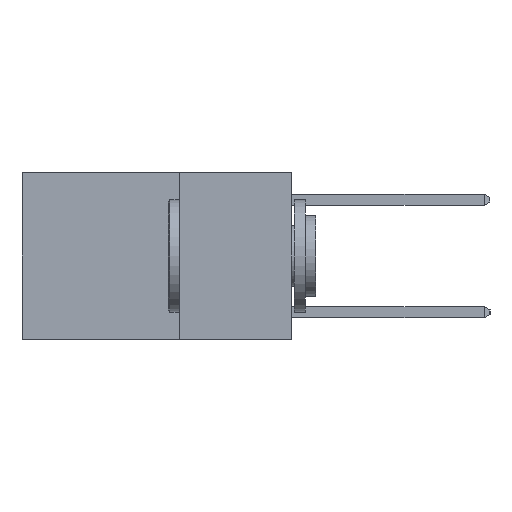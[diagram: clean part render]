
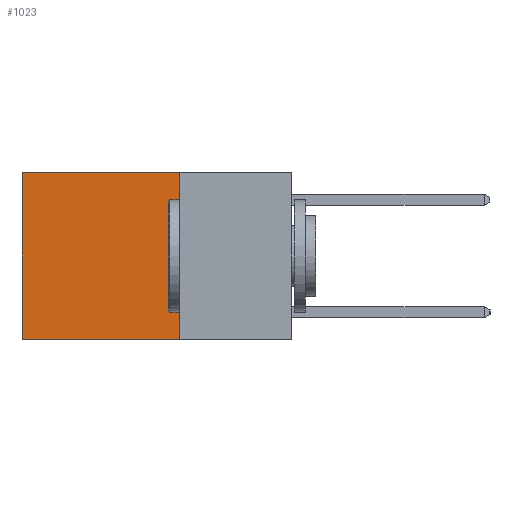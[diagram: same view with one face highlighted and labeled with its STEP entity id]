
A CAD part, left-side view. The second image highlights one B-rep face of the part: STEP entity #1023.
In plain terms, the highlighted planar face has unit normal (-1, 0, 0).
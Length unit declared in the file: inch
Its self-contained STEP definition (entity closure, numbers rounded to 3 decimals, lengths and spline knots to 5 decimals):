
#367 = VECTOR ( 'NONE', #6988, 39.37008 ) ;
#983 = ORIENTED_EDGE ( 'NONE', *, *, #10820, .F. ) ;
#1023 = ADVANCED_FACE ( 'NONE', ( #6357 ), #8432, .F. ) ;
#1138 = DIRECTION ( 'NONE',  ( 0., 0., -1. ) ) ;
#1522 = ORIENTED_EDGE ( 'NONE', *, *, #5323, .F. ) ;
#1647 = CARTESIAN_POINT ( 'NONE',  ( 0.2625, 0.6, -0.37 ) ) ;
#1704 = CARTESIAN_POINT ( 'NONE',  ( 0.2625, 0.6, 0. ) ) ;
#1836 = ORIENTED_EDGE ( 'NONE', *, *, #4123, .T. ) ;
#2904 = CARTESIAN_POINT ( 'NONE',  ( 0.2625, 0.25, 0. ) ) ;
#3054 = CARTESIAN_POINT ( 'NONE',  ( 0.2625, 0.25, 0. ) ) ;
#3218 = VERTEX_POINT ( 'NONE', #5311 ) ;
#3484 = EDGE_LOOP ( 'NONE', ( #4224, #1522, #983, #1836 ) ) ;
#3866 = VECTOR ( 'NONE', #6469, 39.37008 ) ;
#3881 = DIRECTION ( 'NONE',  ( 0., 1., 0. ) ) ;
#4123 = EDGE_CURVE ( 'NONE', #6299, #9887, #9869, .T. ) ;
#4142 = LINE ( 'NONE', #10705, #3866 ) ;
#4224 = ORIENTED_EDGE ( 'NONE', *, *, #5061, .T. ) ;
#4277 = LINE ( 'NONE', #4432, #367 ) ;
#4432 = CARTESIAN_POINT ( 'NONE',  ( 0.2625, 0.6, 0. ) ) ;
#5061 = EDGE_CURVE ( 'NONE', #9887, #5654, #4277, .T. ) ;
#5122 = DIRECTION ( 'NONE',  ( 0., 0., -1. ) ) ;
#5311 = CARTESIAN_POINT ( 'NONE',  ( 0.2625, 0.25, -0.37 ) ) ;
#5323 = EDGE_CURVE ( 'NONE', #3218, #5654, #4142, .T. ) ;
#5654 = VERTEX_POINT ( 'NONE', #1647 ) ;
#6299 = VERTEX_POINT ( 'NONE', #3054 ) ;
#6340 = CARTESIAN_POINT ( 'NONE',  ( 0.2625, 0.25, 0. ) ) ;
#6357 = FACE_OUTER_BOUND ( 'NONE', #3484, .T. ) ;
#6469 = DIRECTION ( 'NONE',  ( 0., 1., 0. ) ) ;
#6988 = DIRECTION ( 'NONE',  ( 0., 0., -1. ) ) ;
#7367 = LINE ( 'NONE', #6340, #9063 ) ;
#7979 = AXIS2_PLACEMENT_3D ( 'NONE', #2904, #9110, #5122 ) ;
#8432 = PLANE ( 'NONE',  #7979 ) ;
#9063 = VECTOR ( 'NONE', #1138, 39.37008 ) ;
#9110 = DIRECTION ( 'NONE',  ( 1., 0., 0. ) ) ;
#9585 = VECTOR ( 'NONE', #3881, 39.37008 ) ;
#9811 = CARTESIAN_POINT ( 'NONE',  ( 0.2625, 0.25, 0. ) ) ;
#9869 = LINE ( 'NONE', #9811, #9585 ) ;
#9887 = VERTEX_POINT ( 'NONE', #1704 ) ;
#10705 = CARTESIAN_POINT ( 'NONE',  ( 0.2625, 0.25, -0.37 ) ) ;
#10820 = EDGE_CURVE ( 'NONE', #6299, #3218, #7367, .T. ) ;
